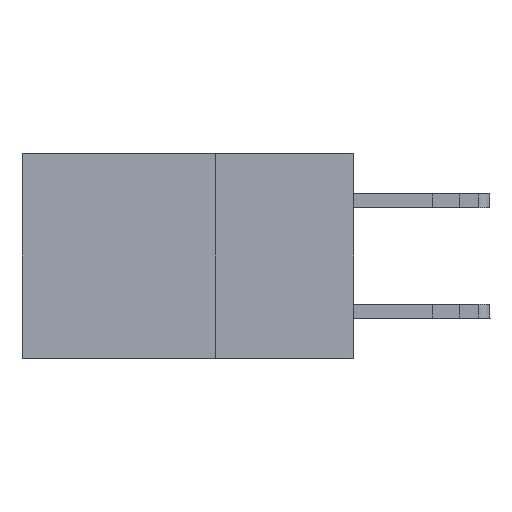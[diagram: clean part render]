
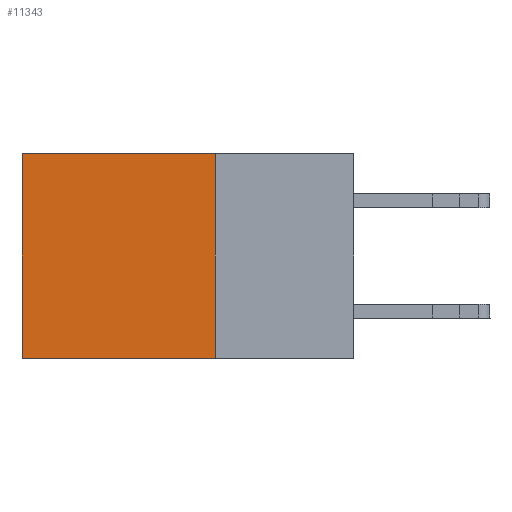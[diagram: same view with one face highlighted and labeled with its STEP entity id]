
A CAD part, left-side view. The second image highlights one B-rep face of the part: STEP entity #11343.
In plain terms, the highlighted planar face has unit normal (-1, 0, 0).
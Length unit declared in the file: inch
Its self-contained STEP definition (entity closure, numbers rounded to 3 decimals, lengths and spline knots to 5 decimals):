
#163 = VERTEX_POINT ( 'NONE', #10362 ) ;
#209 = EDGE_CURVE ( 'NONE', #4969, #163, #7791, .T. ) ;
#252 = CARTESIAN_POINT ( 'NONE',  ( 0.2875, 0.25, 0. ) ) ;
#690 = LINE ( 'NONE', #9358, #2014 ) ;
#1367 = PLANE ( 'NONE',  #9758 ) ;
#1660 = CARTESIAN_POINT ( 'NONE',  ( 0.2875, 0.6, 0. ) ) ;
#1888 = EDGE_CURVE ( 'NONE', #6412, #4969, #3886, .T. ) ;
#2014 = VECTOR ( 'NONE', #5725, 39.37008 ) ;
#3389 = VERTEX_POINT ( 'NONE', #1660 ) ;
#3886 = LINE ( 'NONE', #9896, #11933 ) ;
#3994 = DIRECTION ( 'NONE',  ( 1., 0., 0. ) ) ;
#4258 = VECTOR ( 'NONE', #15144, 39.37008 ) ;
#4969 = VERTEX_POINT ( 'NONE', #10357 ) ;
#4973 = EDGE_LOOP ( 'NONE', ( #11878, #6052, #11399, #5484 ) ) ;
#5158 = DIRECTION ( 'NONE',  ( 0., 0., -1. ) ) ;
#5484 = ORIENTED_EDGE ( 'NONE', *, *, #12145, .T. ) ;
#5725 = DIRECTION ( 'NONE',  ( 0., 1., 0. ) ) ;
#6052 = ORIENTED_EDGE ( 'NONE', *, *, #209, .F. ) ;
#6197 = DIRECTION ( 'NONE',  ( 0., 0., -1. ) ) ;
#6412 = VERTEX_POINT ( 'NONE', #252 ) ;
#7105 = LINE ( 'NONE', #7188, #14526 ) ;
#7188 = CARTESIAN_POINT ( 'NONE',  ( 0.2875, 0.6, 0. ) ) ;
#7791 = LINE ( 'NONE', #11503, #4258 ) ;
#8930 = EDGE_CURVE ( 'NONE', #3389, #163, #7105, .T. ) ;
#9358 = CARTESIAN_POINT ( 'NONE',  ( 0.2875, 0.25, 0. ) ) ;
#9612 = DIRECTION ( 'NONE',  ( 0., 0., -1. ) ) ;
#9758 = AXIS2_PLACEMENT_3D ( 'NONE', #15111, #3994, #5158 ) ;
#9896 = CARTESIAN_POINT ( 'NONE',  ( 0.2875, 0.25, 0. ) ) ;
#10357 = CARTESIAN_POINT ( 'NONE',  ( 0.2875, 0.25, -0.37 ) ) ;
#10362 = CARTESIAN_POINT ( 'NONE',  ( 0.2875, 0.6, -0.37 ) ) ;
#11343 = ADVANCED_FACE ( 'NONE', ( #13670 ), #1367, .F. ) ;
#11399 = ORIENTED_EDGE ( 'NONE', *, *, #1888, .F. ) ;
#11503 = CARTESIAN_POINT ( 'NONE',  ( 0.2875, 0.25, -0.37 ) ) ;
#11878 = ORIENTED_EDGE ( 'NONE', *, *, #8930, .T. ) ;
#11933 = VECTOR ( 'NONE', #6197, 39.37008 ) ;
#12145 = EDGE_CURVE ( 'NONE', #6412, #3389, #690, .T. ) ;
#13670 = FACE_OUTER_BOUND ( 'NONE', #4973, .T. ) ;
#14526 = VECTOR ( 'NONE', #9612, 39.37008 ) ;
#15111 = CARTESIAN_POINT ( 'NONE',  ( 0.2875, 0.25, 0. ) ) ;
#15144 = DIRECTION ( 'NONE',  ( 0., 1., 0. ) ) ;
